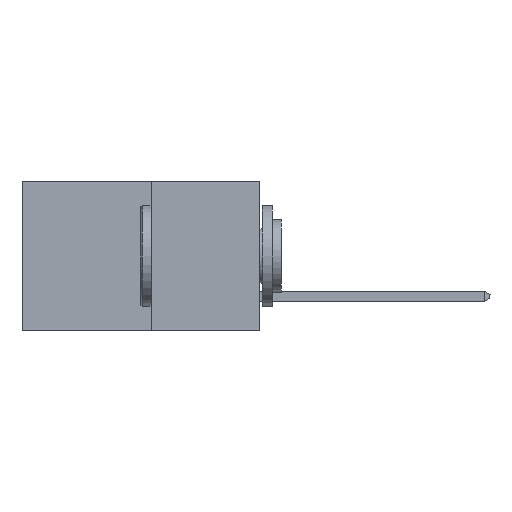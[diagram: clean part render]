
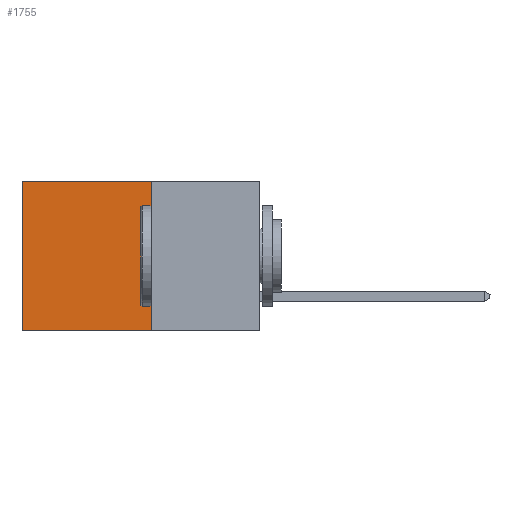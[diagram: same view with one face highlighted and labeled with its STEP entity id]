
A CAD part, left-side view. The second image highlights one B-rep face of the part: STEP entity #1755.
In plain terms, the highlighted planar face has unit normal (-1, 0, 0).
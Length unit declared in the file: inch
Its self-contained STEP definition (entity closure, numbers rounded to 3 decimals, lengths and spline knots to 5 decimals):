
#459 = VECTOR ( 'NONE', #20620, 39.37008 ) ;
#481 = VECTOR ( 'NONE', #20966, 39.37008 ) ;
#1723 = FACE_OUTER_BOUND ( 'NONE', #17754, .T. ) ;
#1755 = ADVANCED_FACE ( 'NONE', ( #1723 ), #24159, .F. ) ;
#2343 = CARTESIAN_POINT ( 'NONE',  ( 0.277, 0.59, 0. ) ) ;
#5219 = LINE ( 'NONE', #8731, #10859 ) ;
#7383 = VERTEX_POINT ( 'NONE', #29497 ) ;
#8412 = DIRECTION ( 'NONE',  ( 0., 0., -1. ) ) ;
#8731 = CARTESIAN_POINT ( 'NONE',  ( 0.277, 0.27, -0.37 ) ) ;
#9476 = CARTESIAN_POINT ( 'NONE',  ( 0.277, 0.27, 0. ) ) ;
#9992 = AXIS2_PLACEMENT_3D ( 'NONE', #23761, #23787, #23652 ) ;
#10859 = VECTOR ( 'NONE', #11170, 39.37008 ) ;
#11170 = DIRECTION ( 'NONE',  ( 0., 1., 0. ) ) ;
#12036 = EDGE_CURVE ( 'NONE', #25784, #13422, #14065, .T. ) ;
#12636 = ORIENTED_EDGE ( 'NONE', *, *, #22887, .F. ) ;
#13422 = VERTEX_POINT ( 'NONE', #2343 ) ;
#13858 = LINE ( 'NONE', #17935, #25810 ) ;
#14065 = LINE ( 'NONE', #18553, #481 ) ;
#17754 = EDGE_LOOP ( 'NONE', ( #24846, #12636, #23504, #21037 ) ) ;
#17935 = CARTESIAN_POINT ( 'NONE',  ( 0.277, 0.27, -0.37 ) ) ;
#18225 = CARTESIAN_POINT ( 'NONE',  ( 0.277, 0.59, -0.37 ) ) ;
#18553 = CARTESIAN_POINT ( 'NONE',  ( 0.277, 0.27, 0. ) ) ;
#20620 = DIRECTION ( 'NONE',  ( 0., 0., -1. ) ) ;
#20966 = DIRECTION ( 'NONE',  ( 0., 1., 0. ) ) ;
#21037 = ORIENTED_EDGE ( 'NONE', *, *, #12036, .T. ) ;
#21408 = CARTESIAN_POINT ( 'NONE',  ( 0.277, 0.59, -0.37 ) ) ;
#22796 = EDGE_CURVE ( 'NONE', #25784, #7383, #13858, .T. ) ;
#22887 = EDGE_CURVE ( 'NONE', #7383, #23830, #5219, .T. ) ;
#23504 = ORIENTED_EDGE ( 'NONE', *, *, #22796, .F. ) ;
#23652 = DIRECTION ( 'NONE',  ( 0., 0., -1. ) ) ;
#23761 = CARTESIAN_POINT ( 'NONE',  ( 0.277, 0.27, -0.37 ) ) ;
#23787 = DIRECTION ( 'NONE',  ( 1., 0., 0. ) ) ;
#23830 = VERTEX_POINT ( 'NONE', #21408 ) ;
#24159 = PLANE ( 'NONE',  #9992 ) ;
#24846 = ORIENTED_EDGE ( 'NONE', *, *, #26233, .T. ) ;
#25784 = VERTEX_POINT ( 'NONE', #9476 ) ;
#25810 = VECTOR ( 'NONE', #8412, 39.37008 ) ;
#26007 = LINE ( 'NONE', #18225, #459 ) ;
#26233 = EDGE_CURVE ( 'NONE', #13422, #23830, #26007, .T. ) ;
#29497 = CARTESIAN_POINT ( 'NONE',  ( 0.277, 0.27, -0.37 ) ) ;
